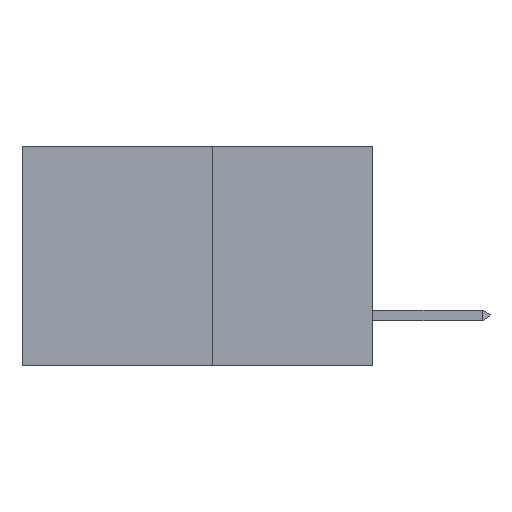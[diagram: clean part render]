
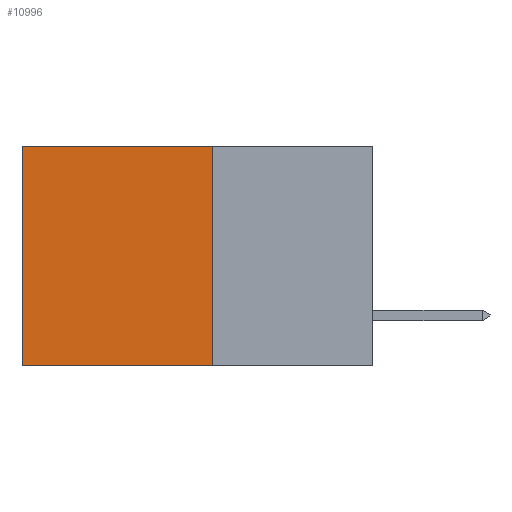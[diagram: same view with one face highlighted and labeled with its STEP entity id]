
A CAD part, left-side view. The second image highlights one B-rep face of the part: STEP entity #10996.
In plain terms, the highlighted planar face has unit normal (-1, 0, 0).
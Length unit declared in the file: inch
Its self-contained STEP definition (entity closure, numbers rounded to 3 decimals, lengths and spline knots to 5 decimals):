
#424 = EDGE_CURVE ( 'NONE', #11618, #712, #8836, .T. ) ;
#712 = VERTEX_POINT ( 'NONE', #11362 ) ;
#1227 = EDGE_CURVE ( 'NONE', #2696, #13858, #3591, .T. ) ;
#1236 = EDGE_CURVE ( 'NONE', #11618, #2696, #9566, .T. ) ;
#1555 = ORIENTED_EDGE ( 'NONE', *, *, #1227, .F. ) ;
#1615 = DIRECTION ( 'NONE',  ( 0., 0., -1. ) ) ;
#1807 = EDGE_CURVE ( 'NONE', #712, #13858, #13298, .T. ) ;
#2696 = VERTEX_POINT ( 'NONE', #11145 ) ;
#3591 = LINE ( 'NONE', #6568, #12758 ) ;
#4926 = ORIENTED_EDGE ( 'NONE', *, *, #424, .T. ) ;
#5346 = AXIS2_PLACEMENT_3D ( 'NONE', #5821, #15340, #8220 ) ;
#5821 = CARTESIAN_POINT ( 'NONE',  ( 0.277, 0.27, -0.37 ) ) ;
#6186 = DIRECTION ( 'NONE',  ( 0., 1., 0. ) ) ;
#6568 = CARTESIAN_POINT ( 'NONE',  ( 0.277, 0.27, -0.37 ) ) ;
#8220 = DIRECTION ( 'NONE',  ( 0., 0., -1. ) ) ;
#8446 = VECTOR ( 'NONE', #6186, 39.37008 ) ;
#8836 = LINE ( 'NONE', #15514, #8446 ) ;
#9181 = VECTOR ( 'NONE', #15332, 39.37008 ) ;
#9347 = VECTOR ( 'NONE', #1615, 39.37008 ) ;
#9566 = LINE ( 'NONE', #13639, #9181 ) ;
#9790 = ORIENTED_EDGE ( 'NONE', *, *, #1236, .F. ) ;
#10454 = DIRECTION ( 'NONE',  ( 0., 1., 0. ) ) ;
#10957 = FACE_OUTER_BOUND ( 'NONE', #13353, .T. ) ;
#10996 = ADVANCED_FACE ( 'NONE', ( #10957 ), #13003, .F. ) ;
#11145 = CARTESIAN_POINT ( 'NONE',  ( 0.277, 0.27, -0.37 ) ) ;
#11362 = CARTESIAN_POINT ( 'NONE',  ( 0.277, 0.59, 0. ) ) ;
#11485 = CARTESIAN_POINT ( 'NONE',  ( 0.277, 0.59, -0.37 ) ) ;
#11618 = VERTEX_POINT ( 'NONE', #11645 ) ;
#11645 = CARTESIAN_POINT ( 'NONE',  ( 0.277, 0.27, 0. ) ) ;
#12758 = VECTOR ( 'NONE', #10454, 39.37008 ) ;
#13003 = PLANE ( 'NONE',  #5346 ) ;
#13298 = LINE ( 'NONE', #11485, #9347 ) ;
#13353 = EDGE_LOOP ( 'NONE', ( #13902, #1555, #9790, #4926 ) ) ;
#13458 = CARTESIAN_POINT ( 'NONE',  ( 0.277, 0.59, -0.37 ) ) ;
#13639 = CARTESIAN_POINT ( 'NONE',  ( 0.277, 0.27, -0.37 ) ) ;
#13858 = VERTEX_POINT ( 'NONE', #13458 ) ;
#13902 = ORIENTED_EDGE ( 'NONE', *, *, #1807, .T. ) ;
#15332 = DIRECTION ( 'NONE',  ( 0., 0., -1. ) ) ;
#15340 = DIRECTION ( 'NONE',  ( 1., 0., 0. ) ) ;
#15514 = CARTESIAN_POINT ( 'NONE',  ( 0.277, 0.27, 0. ) ) ;
